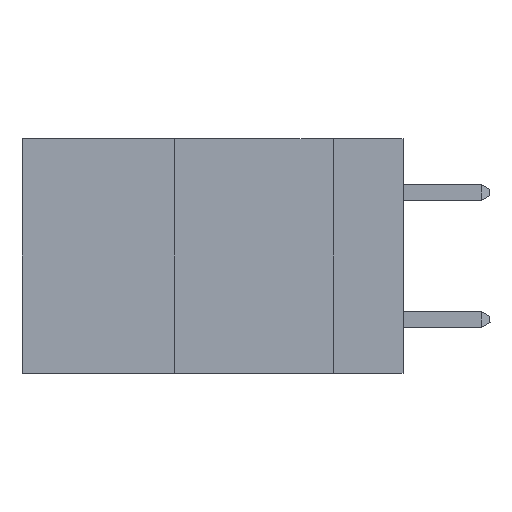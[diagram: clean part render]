
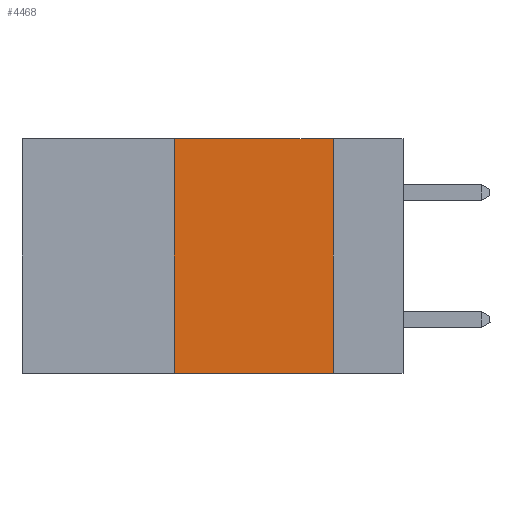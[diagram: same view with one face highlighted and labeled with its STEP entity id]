
A CAD part, left-side view. The second image highlights one B-rep face of the part: STEP entity #4468.
In plain terms, the highlighted planar face has unit normal (-1, 0, 0).
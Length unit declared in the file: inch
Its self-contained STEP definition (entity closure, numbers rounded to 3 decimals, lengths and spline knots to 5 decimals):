
#419 = CARTESIAN_POINT ( 'NONE',  ( 0., 0.11, 0. ) ) ;
#426 = LINE ( 'NONE', #20856, #6453 ) ;
#501 = LINE ( 'NONE', #5835, #3813 ) ;
#1526 = EDGE_CURVE ( 'NONE', #3477, #5890, #426, .T. ) ;
#1596 = ORIENTED_EDGE ( 'NONE', *, *, #12790, .F. ) ;
#1771 = DIRECTION ( 'NONE',  ( 0., -1., 0. ) ) ;
#2706 = DIRECTION ( 'NONE',  ( 0., 0., -1. ) ) ;
#3477 = VERTEX_POINT ( 'NONE', #20144 ) ;
#3813 = VECTOR ( 'NONE', #13427, 39.37008 ) ;
#4280 = EDGE_CURVE ( 'NONE', #15052, #20010, #13150, .T. ) ;
#4468 = ADVANCED_FACE ( 'NONE', ( #12555 ), #4945, .F. ) ;
#4945 = PLANE ( 'NONE',  #12508 ) ;
#5029 = CARTESIAN_POINT ( 'NONE',  ( 0., 0.6, 0. ) ) ;
#5371 = EDGE_LOOP ( 'NONE', ( #1596, #17925, #15403, #20779 ) ) ;
#5835 = CARTESIAN_POINT ( 'NONE',  ( 0., 0.36, 0. ) ) ;
#5890 = VERTEX_POINT ( 'NONE', #11121 ) ;
#6453 = VECTOR ( 'NONE', #1771, 39.37008 ) ;
#10706 = VECTOR ( 'NONE', #2706, 39.37008 ) ;
#10916 = DIRECTION ( 'NONE',  ( 0., 0., -1. ) ) ;
#11121 = CARTESIAN_POINT ( 'NONE',  ( 0., 0.11, -0.37 ) ) ;
#12508 = AXIS2_PLACEMENT_3D ( 'NONE', #5029, #20349, #10916 ) ;
#12555 = FACE_OUTER_BOUND ( 'NONE', #5371, .T. ) ;
#12790 = EDGE_CURVE ( 'NONE', #20010, #5890, #13605, .T. ) ;
#12979 = DIRECTION ( 'NONE',  ( 0., -1., 0. ) ) ;
#13150 = LINE ( 'NONE', #22314, #22680 ) ;
#13427 = DIRECTION ( 'NONE',  ( 0., 0., 1. ) ) ;
#13605 = LINE ( 'NONE', #419, #10706 ) ;
#14810 = CARTESIAN_POINT ( 'NONE',  ( 0., 0.11, 0. ) ) ;
#15052 = VERTEX_POINT ( 'NONE', #21252 ) ;
#15403 = ORIENTED_EDGE ( 'NONE', *, *, #24561, .F. ) ;
#17925 = ORIENTED_EDGE ( 'NONE', *, *, #4280, .F. ) ;
#20010 = VERTEX_POINT ( 'NONE', #14810 ) ;
#20144 = CARTESIAN_POINT ( 'NONE',  ( 0., 0.36, -0.37 ) ) ;
#20349 = DIRECTION ( 'NONE',  ( 1., 0., 0. ) ) ;
#20779 = ORIENTED_EDGE ( 'NONE', *, *, #1526, .T. ) ;
#20856 = CARTESIAN_POINT ( 'NONE',  ( 0., 0.6, -0.37 ) ) ;
#21252 = CARTESIAN_POINT ( 'NONE',  ( 0., 0.36, 0. ) ) ;
#22314 = CARTESIAN_POINT ( 'NONE',  ( 0., 0.6, 0. ) ) ;
#22680 = VECTOR ( 'NONE', #12979, 39.37008 ) ;
#24561 = EDGE_CURVE ( 'NONE', #3477, #15052, #501, .T. ) ;
